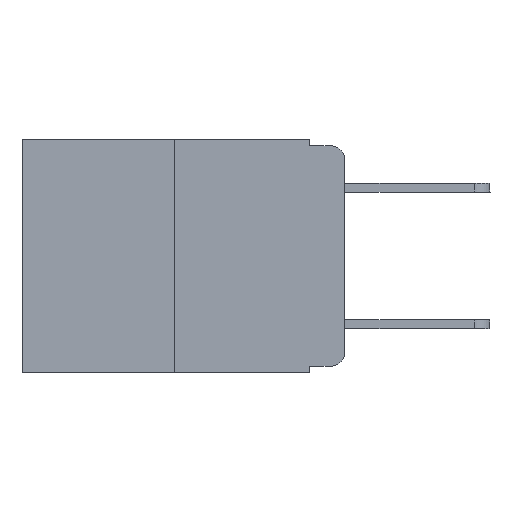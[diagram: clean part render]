
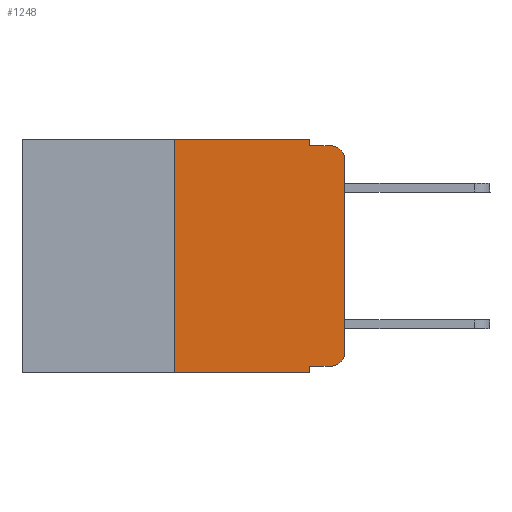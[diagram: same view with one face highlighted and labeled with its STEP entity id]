
A CAD part, left-side view. The second image highlights one B-rep face of the part: STEP entity #1248.
In plain terms, the highlighted planar face has unit normal (-1, 0, 0).
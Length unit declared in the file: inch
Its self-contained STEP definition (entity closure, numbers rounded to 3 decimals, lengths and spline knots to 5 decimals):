
#174 = CARTESIAN_POINT ( 'NONE',  ( 0., 0.02, -0.01 ) ) ;
#519 = VERTEX_POINT ( 'NONE', #6390 ) ;
#1240 = VERTEX_POINT ( 'NONE', #4070 ) ;
#1248 = ADVANCED_FACE ( 'NONE', ( #13009 ), #8086, .F. ) ;
#1299 = EDGE_CURVE ( 'NONE', #1240, #15275, #5857, .T. ) ;
#1391 = CARTESIAN_POINT ( 'NONE',  ( 0., 0.051, -0.343 ) ) ;
#1434 = LINE ( 'NONE', #1955, #16402 ) ;
#1465 = VECTOR ( 'NONE', #7451, 39.37008 ) ;
#1525 = EDGE_CURVE ( 'NONE', #15932, #7150, #7714, .T. ) ;
#1955 = CARTESIAN_POINT ( 'NONE',  ( 0., 0.25, 0. ) ) ;
#2013 = CARTESIAN_POINT ( 'NONE',  ( 0., 0.25, 0. ) ) ;
#2534 = DIRECTION ( 'NONE',  ( 0., -1., 0. ) ) ;
#2670 = VECTOR ( 'NONE', #20017, 39.37008 ) ;
#4070 = CARTESIAN_POINT ( 'NONE',  ( 0., 0., -0.03 ) ) ;
#4918 = LINE ( 'NONE', #12165, #17048 ) ;
#5252 = AXIS2_PLACEMENT_3D ( 'NONE', #23882, #16071, #6339 ) ;
#5549 = LINE ( 'NONE', #20101, #16434 ) ;
#5632 = CARTESIAN_POINT ( 'NONE',  ( 0., 0.051, -0.01 ) ) ;
#5768 = VERTEX_POINT ( 'NONE', #13935 ) ;
#5857 = CIRCLE ( 'NONE', #23068, 0.02 ) ;
#6088 = DIRECTION ( 'NONE',  ( 0., 0., -1. ) ) ;
#6279 = ORIENTED_EDGE ( 'NONE', *, *, #22719, .T. ) ;
#6339 = DIRECTION ( 'NONE',  ( 0., 0., -1. ) ) ;
#6390 = CARTESIAN_POINT ( 'NONE',  ( 0., 0.051, -0.01 ) ) ;
#6558 = ORIENTED_EDGE ( 'NONE', *, *, #7855, .F. ) ;
#6617 = CARTESIAN_POINT ( 'NONE',  ( 0., 0.051, -0.333 ) ) ;
#6958 = EDGE_CURVE ( 'NONE', #20737, #5768, #13642, .T. ) ;
#7150 = VERTEX_POINT ( 'NONE', #10818 ) ;
#7451 = DIRECTION ( 'NONE',  ( 0., 0., -1. ) ) ;
#7714 = LINE ( 'NONE', #6617, #11771 ) ;
#7719 = CARTESIAN_POINT ( 'NONE',  ( 0., 0., -0.313 ) ) ;
#7855 = EDGE_CURVE ( 'NONE', #24257, #20737, #1434, .T. ) ;
#7889 = EDGE_CURVE ( 'NONE', #519, #15275, #19851, .T. ) ;
#8086 = PLANE ( 'NONE',  #20438 ) ;
#8178 = DIRECTION ( 'NONE',  ( 0., 0., 1. ) ) ;
#8304 = CARTESIAN_POINT ( 'NONE',  ( 0., 0.473, -0.343 ) ) ;
#8891 = ORIENTED_EDGE ( 'NONE', *, *, #25759, .F. ) ;
#9255 = ORIENTED_EDGE ( 'NONE', *, *, #14645, .F. ) ;
#9372 = VERTEX_POINT ( 'NONE', #1391 ) ;
#9711 = CARTESIAN_POINT ( 'NONE',  ( 0., 0.051, 0. ) ) ;
#10818 = CARTESIAN_POINT ( 'NONE',  ( 0., 0.02, -0.333 ) ) ;
#11102 = CARTESIAN_POINT ( 'NONE',  ( 0., 0.25, -0.343 ) ) ;
#11246 = CIRCLE ( 'NONE', #5252, 0.02 ) ;
#11771 = VECTOR ( 'NONE', #20531, 39.37008 ) ;
#11797 = VECTOR ( 'NONE', #2534, 39.37008 ) ;
#12007 = CARTESIAN_POINT ( 'NONE',  ( 0., 0.02, -0.03 ) ) ;
#12022 = CARTESIAN_POINT ( 'NONE',  ( 0., 0.051, -0.333 ) ) ;
#12034 = DIRECTION ( 'NONE',  ( 0., -1., 0. ) ) ;
#12165 = CARTESIAN_POINT ( 'NONE',  ( 0., 0.051, 0. ) ) ;
#13009 = FACE_OUTER_BOUND ( 'NONE', #16549, .T. ) ;
#13127 = ORIENTED_EDGE ( 'NONE', *, *, #25256, .T. ) ;
#13642 = LINE ( 'NONE', #14402, #11797 ) ;
#13935 = CARTESIAN_POINT ( 'NONE',  ( 0., 0.051, 0. ) ) ;
#14073 = DIRECTION ( 'NONE',  ( 0., 0., -1. ) ) ;
#14402 = CARTESIAN_POINT ( 'NONE',  ( 0., 0.473, 0. ) ) ;
#14631 = ORIENTED_EDGE ( 'NONE', *, *, #7889, .F. ) ;
#14645 = EDGE_CURVE ( 'NONE', #15932, #9372, #4918, .T. ) ;
#14676 = LINE ( 'NONE', #8304, #16248 ) ;
#15058 = ORIENTED_EDGE ( 'NONE', *, *, #1299, .T. ) ;
#15178 = LINE ( 'NONE', #9711, #1465 ) ;
#15275 = VERTEX_POINT ( 'NONE', #174 ) ;
#15932 = VERTEX_POINT ( 'NONE', #12022 ) ;
#16071 = DIRECTION ( 'NONE',  ( -1., 0., 0. ) ) ;
#16085 = DIRECTION ( 'NONE',  ( -1., 0., 0. ) ) ;
#16248 = VECTOR ( 'NONE', #12034, 39.37008 ) ;
#16402 = VECTOR ( 'NONE', #21636, 39.37008 ) ;
#16434 = VECTOR ( 'NONE', #8178, 39.37008 ) ;
#16549 = EDGE_LOOP ( 'NONE', ( #13127, #15058, #14631, #8891, #23112, #6558, #6279, #9255, #22618, #19891 ) ) ;
#17048 = VECTOR ( 'NONE', #17916, 39.37008 ) ;
#17916 = DIRECTION ( 'NONE',  ( 0., 0., -1. ) ) ;
#18953 = VERTEX_POINT ( 'NONE', #7719 ) ;
#19851 = LINE ( 'NONE', #5632, #2670 ) ;
#19891 = ORIENTED_EDGE ( 'NONE', *, *, #22077, .T. ) ;
#20017 = DIRECTION ( 'NONE',  ( 0., -1., 0. ) ) ;
#20101 = CARTESIAN_POINT ( 'NONE',  ( 0., 0., 0. ) ) ;
#20438 = AXIS2_PLACEMENT_3D ( 'NONE', #21988, #25841, #14073 ) ;
#20531 = DIRECTION ( 'NONE',  ( 0., -1., 0. ) ) ;
#20737 = VERTEX_POINT ( 'NONE', #2013 ) ;
#21636 = DIRECTION ( 'NONE',  ( 0., 0., 1. ) ) ;
#21988 = CARTESIAN_POINT ( 'NONE',  ( 0., 0.473, 0. ) ) ;
#22077 = EDGE_CURVE ( 'NONE', #7150, #18953, #11246, .T. ) ;
#22618 = ORIENTED_EDGE ( 'NONE', *, *, #1525, .T. ) ;
#22719 = EDGE_CURVE ( 'NONE', #24257, #9372, #14676, .T. ) ;
#23068 = AXIS2_PLACEMENT_3D ( 'NONE', #12007, #16085, #6088 ) ;
#23112 = ORIENTED_EDGE ( 'NONE', *, *, #6958, .F. ) ;
#23882 = CARTESIAN_POINT ( 'NONE',  ( 0., 0.02, -0.313 ) ) ;
#24257 = VERTEX_POINT ( 'NONE', #11102 ) ;
#25256 = EDGE_CURVE ( 'NONE', #18953, #1240, #5549, .T. ) ;
#25759 = EDGE_CURVE ( 'NONE', #5768, #519, #15178, .T. ) ;
#25841 = DIRECTION ( 'NONE',  ( 1., 0., 0. ) ) ;
